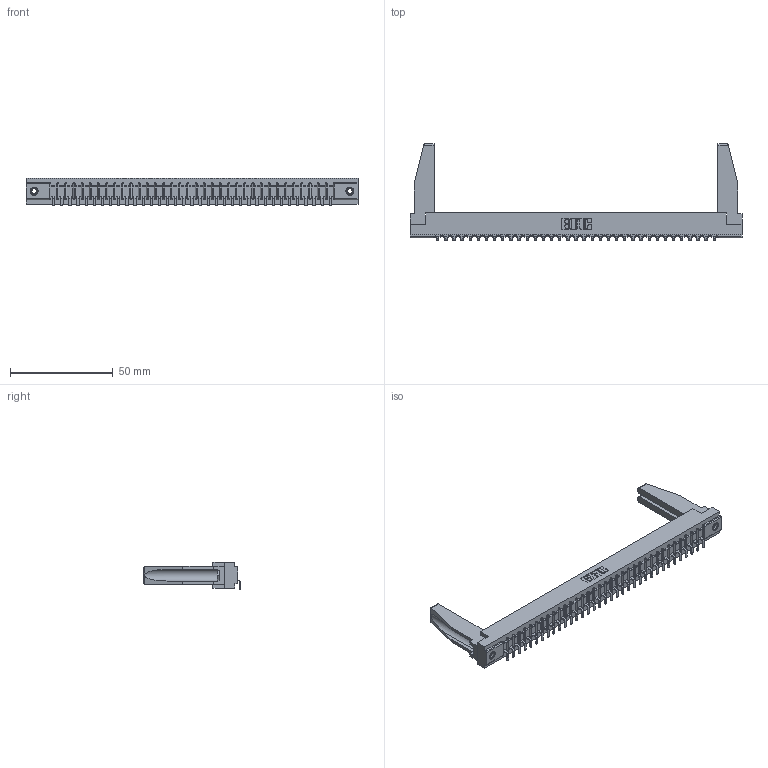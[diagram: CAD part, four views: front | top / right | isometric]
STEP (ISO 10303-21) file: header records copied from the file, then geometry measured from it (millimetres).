
FILE_DESCRIPTION (( 'STEP AP203' ), '1' );
FILE_NAME ('307-035-553-178.STEP', '2019-09-05T07:20:17', ( '' ), ( '' ), 'SwSTEP 2.0', 'SolidWorks 2016', '' );
FILE_SCHEMA (( 'CONFIG_CONTROL_DESIGN' ));
Length unit declared in the file: inch
Products named in the file (5): 307-220-078; 307-290-002_553; 345-250-001_345-250-001-102; 307-035-553-178; 307 Part_.156 Dia Mounting Holes
Assembly tree (40 placements, depth 2):
  307-035-553-178
    307 Part_.156 Dia Mounting Holes
    307-290-002_553  x35
    307-220-078  x2
    345-250-001_345-250-001-102  x2
Bounding box: 161.7 x 47.03 x 13.5 mm (x, y, z)
Volume: 21244.5 mm3; surface area: 25357.2 mm2
Topology: 40 solids, 40 shells, 3014 faces, 9193 edges, 6022 vertices
Faces by surface type: plane 1799, cylinder 1127, sphere 72, cone 12, torus 4
Entity records: 34161 total; most frequent: CARTESIAN_POINT 5762, ORIENTED_EDGE 5708, DIRECTION 5558, EDGE_CURVE 2854, VECTOR 2186, LINE 2186, VERTEX_POINT 1848, AXIS2_PLACEMENT_3D 1686
